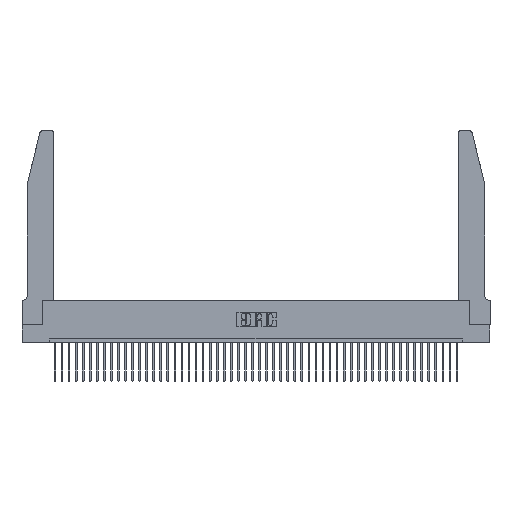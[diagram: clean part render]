
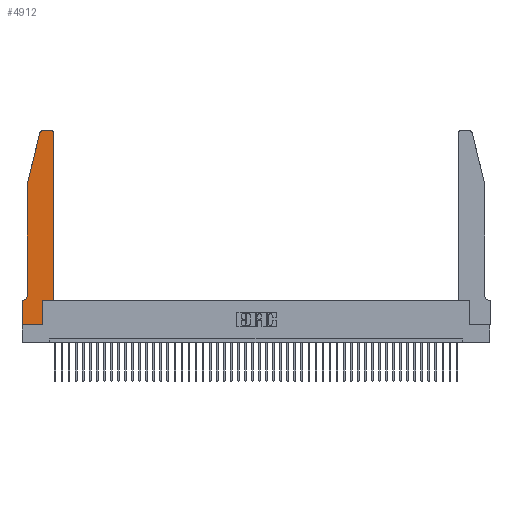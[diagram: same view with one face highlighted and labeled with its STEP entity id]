
A CAD part, top view. The second image highlights one B-rep face of the part: STEP entity #4912.
In plain terms, the highlighted planar face has unit normal (0, 0, 1).
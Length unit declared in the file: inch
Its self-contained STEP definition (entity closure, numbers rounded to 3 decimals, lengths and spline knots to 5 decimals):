
#1341 = CARTESIAN_POINT ( 'NONE',  ( 0.0055, 0.35, 0.37 ) ) ;
#2065 = CARTESIAN_POINT ( 'NONE',  ( 0.25487, 2.72718, 0.37 ) ) ;
#2603 = EDGE_CURVE ( 'NONE', #3993, #32388, #12467, .T. ) ;
#3993 = VERTEX_POINT ( 'NONE', #1341 ) ;
#4075 = DIRECTION ( 'NONE',  ( -1., 0., 0. ) ) ;
#4262 = VERTEX_POINT ( 'NONE', #12103 ) ;
#4455 = LINE ( 'NONE', #25271, #27443 ) ;
#4912 = ADVANCED_FACE ( 'NONE', ( #15024 ), #36242, .T. ) ;
#4975 = LINE ( 'NONE', #37129, #35178 ) ;
#5219 = LINE ( 'NONE', #17780, #16429 ) ;
#5543 = VERTEX_POINT ( 'NONE', #11403 ) ;
#5745 = VECTOR ( 'NONE', #32104, 39.37008 ) ;
#6485 = CARTESIAN_POINT ( 'NONE',  ( 0., 0., 0.37 ) ) ;
#6704 = ORIENTED_EDGE ( 'NONE', *, *, #2603, .T. ) ;
#6970 = CIRCLE ( 'NONE', #7249, 0.03 ) ;
#7241 = LINE ( 'NONE', #33727, #38029 ) ;
#7249 = AXIS2_PLACEMENT_3D ( 'NONE', #12854, #30081, #26513 ) ;
#9531 = ORIENTED_EDGE ( 'NONE', *, *, #18502, .T. ) ;
#10155 = VERTEX_POINT ( 'NONE', #39197 ) ;
#10351 = CARTESIAN_POINT ( 'NONE',  ( 0.0755, 0.35, 0.37 ) ) ;
#10759 = VECTOR ( 'NONE', #4075, 39.37008 ) ;
#11403 = CARTESIAN_POINT ( 'NONE',  ( 0.284, 2.75, 0.37 ) ) ;
#11882 = EDGE_CURVE ( 'NONE', #26712, #4262, #4975, .T. ) ;
#12103 = CARTESIAN_POINT ( 'NONE',  ( 0.4505, 0.35, 0.37 ) ) ;
#12467 = LINE ( 'NONE', #10351, #5745 ) ;
#12577 = EDGE_CURVE ( 'NONE', #14860, #21420, #31954, .T. ) ;
#12772 = AXIS2_PLACEMENT_3D ( 'NONE', #38900, #25750, #39048 ) ;
#12854 = CARTESIAN_POINT ( 'NONE',  ( 0.284, 2.72, 0.37 ) ) ;
#12857 = VERTEX_POINT ( 'NONE', #44243 ) ;
#14860 = VERTEX_POINT ( 'NONE', #2065 ) ;
#15024 = FACE_OUTER_BOUND ( 'NONE', #30307, .T. ) ;
#15341 = DIRECTION ( 'NONE',  ( 0., 0., 1. ) ) ;
#15354 = CARTESIAN_POINT ( 'NONE',  ( 0., 0.35, 0.37 ) ) ;
#15807 = LINE ( 'NONE', #29677, #10759 ) ;
#16429 = VECTOR ( 'NONE', #32723, 39.37008 ) ;
#16773 = DIRECTION ( 'NONE',  ( -1., 0., 0. ) ) ;
#17108 = VECTOR ( 'NONE', #18438, 39.37008 ) ;
#17328 = VECTOR ( 'NONE', #42661, 39.37008 ) ;
#17479 = AXIS2_PLACEMENT_3D ( 'NONE', #34601, #38330, #16773 ) ;
#17780 = CARTESIAN_POINT ( 'NONE',  ( 0.4505, 0.35, 0.37 ) ) ;
#17838 = AXIS2_PLACEMENT_3D ( 'NONE', #29907, #15341, #44296 ) ;
#18286 = CIRCLE ( 'NONE', #17838, 0.03 ) ;
#18438 = DIRECTION ( 'NONE',  ( 0., -1., 0. ) ) ;
#18502 = EDGE_CURVE ( 'NONE', #32388, #32553, #27460, .T. ) ;
#18976 = DIRECTION ( 'NONE',  ( 1., 0., 0. ) ) ;
#19327 = CIRCLE ( 'NONE', #17479, 0.07 ) ;
#19344 = EDGE_CURVE ( 'NONE', #33594, #23512, #18286, .T. ) ;
#19841 = CARTESIAN_POINT ( 'NONE',  ( 0.2865, 0.35, 0.37 ) ) ;
#21420 = VERTEX_POINT ( 'NONE', #37543 ) ;
#22513 = CARTESIAN_POINT ( 'NONE',  ( 0.0755, 2., 0.37 ) ) ;
#23512 = VERTEX_POINT ( 'NONE', #38396 ) ;
#23668 = EDGE_CURVE ( 'NONE', #12857, #26712, #4455, .T. ) ;
#24213 = EDGE_CURVE ( 'NONE', #32553, #12857, #7241, .T. ) ;
#24392 = LINE ( 'NONE', #43116, #17108 ) ;
#24734 = CARTESIAN_POINT ( 'NONE',  ( 0., 0., 0.37 ) ) ;
#25271 = CARTESIAN_POINT ( 'NONE',  ( 0.2865, 0.35, 0.37 ) ) ;
#25750 = DIRECTION ( 'NONE',  ( 0., 0., 1. ) ) ;
#26513 = DIRECTION ( 'NONE',  ( 1., 0., 0. ) ) ;
#26712 = VERTEX_POINT ( 'NONE', #19841 ) ;
#26715 = ORIENTED_EDGE ( 'NONE', *, *, #32393, .T. ) ;
#26881 = ORIENTED_EDGE ( 'NONE', *, *, #24213, .T. ) ;
#27110 = ORIENTED_EDGE ( 'NONE', *, *, #33051, .T. ) ;
#27443 = VECTOR ( 'NONE', #33082, 39.37008 ) ;
#27460 = LINE ( 'NONE', #24734, #17328 ) ;
#28315 = EDGE_CURVE ( 'NONE', #23512, #5543, #15807, .T. ) ;
#28388 = ORIENTED_EDGE ( 'NONE', *, *, #11882, .T. ) ;
#29189 = ORIENTED_EDGE ( 'NONE', *, *, #12577, .T. ) ;
#29677 = CARTESIAN_POINT ( 'NONE',  ( 0.2605, 2.75, 0.37 ) ) ;
#29907 = CARTESIAN_POINT ( 'NONE',  ( 0.4205, 2.72, 0.37 ) ) ;
#30081 = DIRECTION ( 'NONE',  ( 0., 0., 1. ) ) ;
#30307 = EDGE_LOOP ( 'NONE', ( #36457, #26715, #29189, #40406, #45034, #6704, #9531, #26881, #36021, #28388, #27110, #32815 ) ) ;
#30342 = DIRECTION ( 'NONE',  ( -0.239, -0.971, 0. ) ) ;
#30729 = DIRECTION ( 'NONE',  ( 1., 0., 0. ) ) ;
#31954 = LINE ( 'NONE', #22513, #34644 ) ;
#32104 = DIRECTION ( 'NONE',  ( -1., 0., 0. ) ) ;
#32388 = VERTEX_POINT ( 'NONE', #15354 ) ;
#32393 = EDGE_CURVE ( 'NONE', #5543, #14860, #6970, .T. ) ;
#32553 = VERTEX_POINT ( 'NONE', #6485 ) ;
#32723 = DIRECTION ( 'NONE',  ( 0., 1., 0. ) ) ;
#32815 = ORIENTED_EDGE ( 'NONE', *, *, #19344, .T. ) ;
#33051 = EDGE_CURVE ( 'NONE', #4262, #33594, #5219, .T. ) ;
#33082 = DIRECTION ( 'NONE',  ( 0., 1., 0. ) ) ;
#33594 = VERTEX_POINT ( 'NONE', #36605 ) ;
#33727 = CARTESIAN_POINT ( 'NONE',  ( 0., 0., 0.37 ) ) ;
#34601 = CARTESIAN_POINT ( 'NONE',  ( 0.0055, 0.42, 0.37 ) ) ;
#34644 = VECTOR ( 'NONE', #30342, 39.37008 ) ;
#35178 = VECTOR ( 'NONE', #30729, 39.37008 ) ;
#36021 = ORIENTED_EDGE ( 'NONE', *, *, #23668, .T. ) ;
#36242 = PLANE ( 'NONE',  #12772 ) ;
#36457 = ORIENTED_EDGE ( 'NONE', *, *, #28315, .T. ) ;
#36605 = CARTESIAN_POINT ( 'NONE',  ( 0.4505, 2.72, 0.37 ) ) ;
#37129 = CARTESIAN_POINT ( 'NONE',  ( 0.4505, 0.35, 0.37 ) ) ;
#37543 = CARTESIAN_POINT ( 'NONE',  ( 0.0755, 2., 0.37 ) ) ;
#38029 = VECTOR ( 'NONE', #18976, 39.37008 ) ;
#38330 = DIRECTION ( 'NONE',  ( 0., 0., -1. ) ) ;
#38396 = CARTESIAN_POINT ( 'NONE',  ( 0.4205, 2.75, 0.37 ) ) ;
#38900 = CARTESIAN_POINT ( 'NONE',  ( 0., 0.35, 0.37 ) ) ;
#39048 = DIRECTION ( 'NONE',  ( 1., 0., 0. ) ) ;
#39197 = CARTESIAN_POINT ( 'NONE',  ( 0.0755, 0.42, 0.37 ) ) ;
#40406 = ORIENTED_EDGE ( 'NONE', *, *, #43138, .T. ) ;
#42661 = DIRECTION ( 'NONE',  ( 0., -1., 0. ) ) ;
#42916 = EDGE_CURVE ( 'NONE', #10155, #3993, #19327, .T. ) ;
#43116 = CARTESIAN_POINT ( 'NONE',  ( 0.0755, 2., 0.37 ) ) ;
#43138 = EDGE_CURVE ( 'NONE', #21420, #10155, #24392, .T. ) ;
#44243 = CARTESIAN_POINT ( 'NONE',  ( 0.2865, 0., 0.37 ) ) ;
#44296 = DIRECTION ( 'NONE',  ( 1., 0., 0. ) ) ;
#45034 = ORIENTED_EDGE ( 'NONE', *, *, #42916, .T. ) ;
